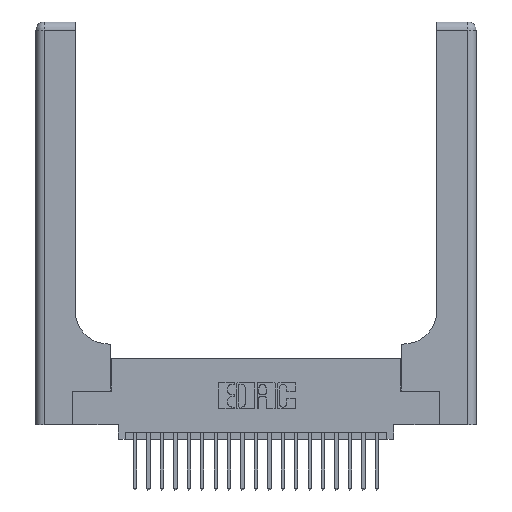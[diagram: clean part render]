
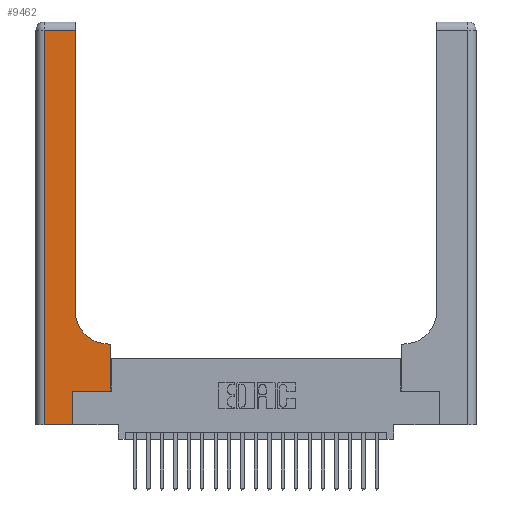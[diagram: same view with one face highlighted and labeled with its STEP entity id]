
A CAD part, top view. The second image highlights one B-rep face of the part: STEP entity #9462.
In plain terms, the highlighted planar face has unit normal (0, 0, 1).
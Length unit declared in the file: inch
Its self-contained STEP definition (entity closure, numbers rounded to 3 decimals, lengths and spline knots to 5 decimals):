
#135 = AXIS2_PLACEMENT_3D ( 'NONE', #1993, #7767, #11119 ) ;
#718 = EDGE_LOOP ( 'NONE', ( #23080, #23159, #17261, #17356, #17647, #17245, #5607, #20975, #21421 ) ) ;
#867 = DIRECTION ( 'NONE',  ( 0., -1., 0. ) ) ;
#1166 = FACE_OUTER_BOUND ( 'NONE', #718, .T. ) ;
#1270 = VECTOR ( 'NONE', #18492, 39.37008 ) ;
#1393 = CARTESIAN_POINT ( 'NONE',  ( 0.2915, 0.6, 0.37 ) ) ;
#1765 = CARTESIAN_POINT ( 'NONE',  ( 0.269, 0.25, 0.37 ) ) ;
#1976 = CARTESIAN_POINT ( 'NONE',  ( 0.2915, 3., 0.37 ) ) ;
#1993 = CARTESIAN_POINT ( 'NONE',  ( 0.5415, 0.85, 0.37 ) ) ;
#2008 = VECTOR ( 'NONE', #6964, 39.37008 ) ;
#2279 = AXIS2_PLACEMENT_3D ( 'NONE', #15554, #6556, #22757 ) ;
#2444 = EDGE_CURVE ( 'NONE', #9046, #7422, #12488, .T. ) ;
#2763 = EDGE_CURVE ( 'NONE', #10423, #12703, #2824, .T. ) ;
#2802 = VECTOR ( 'NONE', #10704, 39.37008 ) ;
#2824 = LINE ( 'NONE', #7534, #10487 ) ;
#3060 = CARTESIAN_POINT ( 'NONE',  ( 0.2915, 2.94, 0.37 ) ) ;
#4343 = VERTEX_POINT ( 'NONE', #16340 ) ;
#4526 = CIRCLE ( 'NONE', #135, 0.25 ) ;
#4613 = EDGE_CURVE ( 'NONE', #20089, #8373, #8437, .T. ) ;
#5013 = VECTOR ( 'NONE', #12032, 39.37008 ) ;
#5607 = ORIENTED_EDGE ( 'NONE', *, *, #22531, .T. ) ;
#6370 = EDGE_CURVE ( 'NONE', #12703, #20207, #19611, .T. ) ;
#6556 = DIRECTION ( 'NONE',  ( 0., 0., -1. ) ) ;
#6927 = CARTESIAN_POINT ( 'NONE',  ( 0.269, 0.25, 0.37 ) ) ;
#6964 = DIRECTION ( 'NONE',  ( -1., 0., 0. ) ) ;
#7214 = CARTESIAN_POINT ( 'NONE',  ( 0.5585, 0.6, 0.37 ) ) ;
#7237 = LINE ( 'NONE', #9836, #1270 ) ;
#7414 = CARTESIAN_POINT ( 'NONE',  ( 0.06, 2.94, 0.37 ) ) ;
#7422 = VERTEX_POINT ( 'NONE', #15760 ) ;
#7433 = CARTESIAN_POINT ( 'NONE',  ( 0.5585, 0.25, 0.37 ) ) ;
#7534 = CARTESIAN_POINT ( 'NONE',  ( 0.06, 3., 0.37 ) ) ;
#7666 = VECTOR ( 'NONE', #12233, 39.37008 ) ;
#7675 = LINE ( 'NONE', #10448, #2008 ) ;
#7767 = DIRECTION ( 'NONE',  ( 0., 0., -1. ) ) ;
#8373 = VERTEX_POINT ( 'NONE', #19285 ) ;
#8437 = LINE ( 'NONE', #1393, #5013 ) ;
#9046 = VERTEX_POINT ( 'NONE', #1765 ) ;
#9462 = ADVANCED_FACE ( 'NONE', ( #1166 ), #22674, .F. ) ;
#9733 = CARTESIAN_POINT ( 'NONE',  ( 0.269, 0., 0.37 ) ) ;
#9836 = CARTESIAN_POINT ( 'NONE',  ( 0.269, 0., 0.37 ) ) ;
#10423 = VERTEX_POINT ( 'NONE', #7414 ) ;
#10448 = CARTESIAN_POINT ( 'NONE',  ( 0., 2.94, 0.37 ) ) ;
#10487 = VECTOR ( 'NONE', #867, 39.37008 ) ;
#10704 = DIRECTION ( 'NONE',  ( 0., 1., 0. ) ) ;
#10996 = DIRECTION ( 'NONE',  ( 0., 1., 0. ) ) ;
#11119 = DIRECTION ( 'NONE',  ( 1., 0., 0. ) ) ;
#11171 = EDGE_CURVE ( 'NONE', #20207, #9046, #7237, .T. ) ;
#12032 = DIRECTION ( 'NONE',  ( -1., 0., 0. ) ) ;
#12233 = DIRECTION ( 'NONE',  ( 1., 0., 0. ) ) ;
#12488 = LINE ( 'NONE', #6927, #7666 ) ;
#12526 = CARTESIAN_POINT ( 'NONE',  ( 0., 0., 0.37 ) ) ;
#12703 = VERTEX_POINT ( 'NONE', #19121 ) ;
#14037 = EDGE_CURVE ( 'NONE', #22874, #10423, #7675, .T. ) ;
#14326 = DIRECTION ( 'NONE',  ( 1., 0., 0. ) ) ;
#15554 = CARTESIAN_POINT ( 'NONE',  ( 0., 3., 0.37 ) ) ;
#15688 = VECTOR ( 'NONE', #14326, 39.37008 ) ;
#15760 = CARTESIAN_POINT ( 'NONE',  ( 0.5585, 0.25, 0.37 ) ) ;
#16340 = CARTESIAN_POINT ( 'NONE',  ( 0.2915, 0.85, 0.37 ) ) ;
#17106 = LINE ( 'NONE', #7433, #21286 ) ;
#17245 = ORIENTED_EDGE ( 'NONE', *, *, #2444, .T. ) ;
#17261 = ORIENTED_EDGE ( 'NONE', *, *, #2763, .T. ) ;
#17356 = ORIENTED_EDGE ( 'NONE', *, *, #6370, .T. ) ;
#17647 = ORIENTED_EDGE ( 'NONE', *, *, #11171, .T. ) ;
#18492 = DIRECTION ( 'NONE',  ( 0., 1., 0. ) ) ;
#18854 = EDGE_CURVE ( 'NONE', #8373, #4343, #4526, .T. ) ;
#19121 = CARTESIAN_POINT ( 'NONE',  ( 0.06, 0., 0.37 ) ) ;
#19285 = CARTESIAN_POINT ( 'NONE',  ( 0.5415, 0.6, 0.37 ) ) ;
#19430 = LINE ( 'NONE', #1976, #2802 ) ;
#19611 = LINE ( 'NONE', #12526, #15688 ) ;
#20016 = EDGE_CURVE ( 'NONE', #4343, #22874, #19430, .T. ) ;
#20089 = VERTEX_POINT ( 'NONE', #7214 ) ;
#20207 = VERTEX_POINT ( 'NONE', #9733 ) ;
#20975 = ORIENTED_EDGE ( 'NONE', *, *, #4613, .T. ) ;
#21286 = VECTOR ( 'NONE', #10996, 39.37008 ) ;
#21421 = ORIENTED_EDGE ( 'NONE', *, *, #18854, .T. ) ;
#22531 = EDGE_CURVE ( 'NONE', #7422, #20089, #17106, .T. ) ;
#22674 = PLANE ( 'NONE',  #2279 ) ;
#22757 = DIRECTION ( 'NONE',  ( -1., 0., 0. ) ) ;
#22874 = VERTEX_POINT ( 'NONE', #3060 ) ;
#23080 = ORIENTED_EDGE ( 'NONE', *, *, #20016, .T. ) ;
#23159 = ORIENTED_EDGE ( 'NONE', *, *, #14037, .T. ) ;
